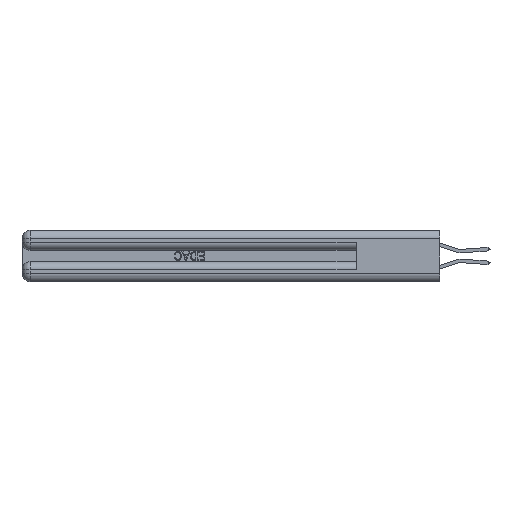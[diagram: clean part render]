
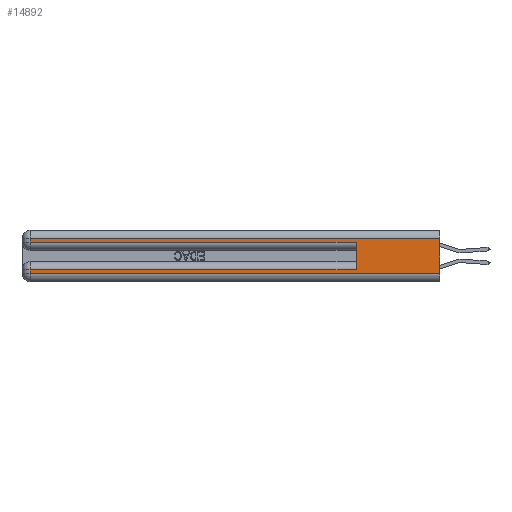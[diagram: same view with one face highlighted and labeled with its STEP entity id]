
A CAD part, left-side view. The second image highlights one B-rep face of the part: STEP entity #14892.
In plain terms, the highlighted planar face has unit normal (-1, 0, 0).
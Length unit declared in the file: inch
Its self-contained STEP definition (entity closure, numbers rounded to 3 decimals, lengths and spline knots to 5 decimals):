
#429 = VECTOR ( 'NONE', #34242, 39.37008 ) ;
#1153 = EDGE_CURVE ( 'NONE', #15432, #6522, #38423, .T. ) ;
#2021 = EDGE_CURVE ( 'NONE', #17176, #40422, #5924, .T. ) ;
#3723 = ORIENTED_EDGE ( 'NONE', *, *, #1153, .F. ) ;
#4488 = CARTESIAN_POINT ( 'NONE',  ( 0., 0., 0.37 ) ) ;
#5279 = EDGE_CURVE ( 'NONE', #18626, #6522, #28359, .T. ) ;
#5352 = CARTESIAN_POINT ( 'NONE',  ( 0., 0., 0.31 ) ) ;
#5924 = LINE ( 'NONE', #36269, #43246 ) ;
#6522 = VERTEX_POINT ( 'NONE', #44475 ) ;
#6658 = ORIENTED_EDGE ( 'NONE', *, *, #14447, .T. ) ;
#6922 = CARTESIAN_POINT ( 'NONE',  ( 0., 0., 0.06 ) ) ;
#6947 = LINE ( 'NONE', #23254, #429 ) ;
#7675 = DIRECTION ( 'NONE',  ( 0., 1., 0. ) ) ;
#9822 = DIRECTION ( 'NONE',  ( 0., 0., -1. ) ) ;
#11218 = VECTOR ( 'NONE', #7675, 39.37008 ) ;
#13110 = CARTESIAN_POINT ( 'NONE',  ( 0., 2.94, 0.31 ) ) ;
#13241 = VECTOR ( 'NONE', #29659, 39.37008 ) ;
#14447 = EDGE_CURVE ( 'NONE', #15432, #26732, #40482, .T. ) ;
#14892 = ADVANCED_FACE ( 'NONE', ( #29637 ), #42775, .F. ) ;
#15432 = VERTEX_POINT ( 'NONE', #19661 ) ;
#15925 = CARTESIAN_POINT ( 'NONE',  ( 0., 0., 0.285 ) ) ;
#16292 = CARTESIAN_POINT ( 'NONE',  ( 0., 0.6, 0.145 ) ) ;
#16590 = DIRECTION ( 'NONE',  ( 0., 0., 1. ) ) ;
#17176 = VERTEX_POINT ( 'NONE', #5352 ) ;
#18325 = CARTESIAN_POINT ( 'NONE',  ( 0., 0., 0.06 ) ) ;
#18406 = DIRECTION ( 'NONE',  ( 0., 0., -1. ) ) ;
#18626 = VERTEX_POINT ( 'NONE', #43431 ) ;
#19661 = CARTESIAN_POINT ( 'NONE',  ( 0., 0.6, 0.085 ) ) ;
#20591 = CARTESIAN_POINT ( 'NONE',  ( 0., 2.94, 0.085 ) ) ;
#20637 = VECTOR ( 'NONE', #9822, 39.37008 ) ;
#23254 = CARTESIAN_POINT ( 'NONE',  ( 0., 0., 0.31 ) ) ;
#23376 = EDGE_CURVE ( 'NONE', #29222, #18626, #35812, .T. ) ;
#24133 = LINE ( 'NONE', #6922, #37644 ) ;
#25309 = AXIS2_PLACEMENT_3D ( 'NONE', #4488, #42304, #18406 ) ;
#25473 = EDGE_CURVE ( 'NONE', #35013, #40422, #24133, .T. ) ;
#26732 = VERTEX_POINT ( 'NONE', #20591 ) ;
#26819 = EDGE_CURVE ( 'NONE', #26732, #35013, #30021, .T. ) ;
#27659 = CARTESIAN_POINT ( 'NONE',  ( 0., 2.94, 0.37 ) ) ;
#27809 = VECTOR ( 'NONE', #37528, 39.37008 ) ;
#28119 = VECTOR ( 'NONE', #16590, 39.37008 ) ;
#28229 = CARTESIAN_POINT ( 'NONE',  ( 0., 0., 0.085 ) ) ;
#28359 = LINE ( 'NONE', #15925, #13241 ) ;
#29222 = VERTEX_POINT ( 'NONE', #13110 ) ;
#29258 = ORIENTED_EDGE ( 'NONE', *, *, #23376, .T. ) ;
#29637 = FACE_OUTER_BOUND ( 'NONE', #42144, .T. ) ;
#29659 = DIRECTION ( 'NONE',  ( 0., -1., 0. ) ) ;
#30021 = LINE ( 'NONE', #40722, #27809 ) ;
#31132 = DIRECTION ( 'NONE',  ( 0., -1., 0. ) ) ;
#31312 = ORIENTED_EDGE ( 'NONE', *, *, #26819, .T. ) ;
#31491 = CARTESIAN_POINT ( 'NONE',  ( 0., 2.94, 0.06 ) ) ;
#34242 = DIRECTION ( 'NONE',  ( 0., 1., 0. ) ) ;
#34676 = ORIENTED_EDGE ( 'NONE', *, *, #5279, .T. ) ;
#35013 = VERTEX_POINT ( 'NONE', #31491 ) ;
#35812 = LINE ( 'NONE', #27659, #20637 ) ;
#36269 = CARTESIAN_POINT ( 'NONE',  ( 0., 0., 0.37 ) ) ;
#36418 = DIRECTION ( 'NONE',  ( 0., 0., -1. ) ) ;
#37528 = DIRECTION ( 'NONE',  ( 0., 0., -1. ) ) ;
#37644 = VECTOR ( 'NONE', #31132, 39.37008 ) ;
#37657 = ORIENTED_EDGE ( 'NONE', *, *, #2021, .F. ) ;
#38423 = LINE ( 'NONE', #16292, #28119 ) ;
#38753 = EDGE_CURVE ( 'NONE', #17176, #29222, #6947, .T. ) ;
#40422 = VERTEX_POINT ( 'NONE', #18325 ) ;
#40482 = LINE ( 'NONE', #28229, #11218 ) ;
#40722 = CARTESIAN_POINT ( 'NONE',  ( 0., 2.94, 0.37 ) ) ;
#41181 = ORIENTED_EDGE ( 'NONE', *, *, #25473, .T. ) ;
#42144 = EDGE_LOOP ( 'NONE', ( #37657, #44393, #29258, #34676, #3723, #6658, #31312, #41181 ) ) ;
#42304 = DIRECTION ( 'NONE',  ( 1., 0., 0. ) ) ;
#42775 = PLANE ( 'NONE',  #25309 ) ;
#43246 = VECTOR ( 'NONE', #36418, 39.37008 ) ;
#43431 = CARTESIAN_POINT ( 'NONE',  ( 0., 2.94, 0.285 ) ) ;
#44393 = ORIENTED_EDGE ( 'NONE', *, *, #38753, .T. ) ;
#44475 = CARTESIAN_POINT ( 'NONE',  ( 0., 0.6, 0.285 ) ) ;
